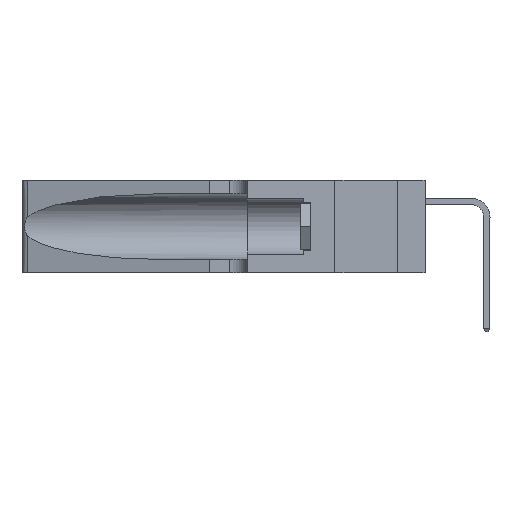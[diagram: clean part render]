
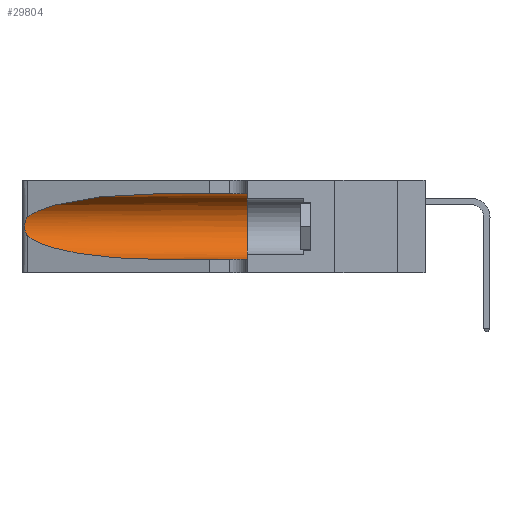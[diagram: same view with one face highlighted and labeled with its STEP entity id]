
A CAD part, left-side view. The second image highlights one B-rep face of the part: STEP entity #29804.
In plain terms, the highlighted cylindrical face has radius 3.308 mm (diameter 6.617 mm), a partial arc.
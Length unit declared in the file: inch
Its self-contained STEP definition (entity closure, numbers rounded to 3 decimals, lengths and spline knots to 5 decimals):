
#890 = EDGE_LOOP ( 'NONE', ( #8014, #15814, #40737, #19634, #7683, #2718 ) ) ;
#2718 = ORIENTED_EDGE ( 'NONE', *, *, #32880, .F. ) ;
#2881 = CARTESIAN_POINT ( 'NONE',  ( 0.25854, 1.2359, 0.20912 ) ) ;
#5132 = DIRECTION ( 'NONE',  ( 0., 1., 0. ) ) ;
#5824 = B_SPLINE_CURVE_WITH_KNOTS ( 'NONE', 3,
 ( #31138, #12391, #40559, #21838, #2881, #24994, #6144, #28142, #9344, #31278, #12522, #34421, #15643, #37551 ),
 .UNSPECIFIED., .F., .F.,
 ( 4, 2, 2, 2, 2, 2, 4 ),
 ( 0., 0.00027, 0.00053, 0.00107, 0.0016, 0.00187, 0.00214 ),
 .UNSPECIFIED. ) ;
#6144 = CARTESIAN_POINT ( 'NONE',  ( 0.26075, 1.23896, 0.19203 ) ) ;
#6509 = CARTESIAN_POINT ( 'NONE',  ( 0.1305, 0.72297, 0.31525 ) ) ;
#7683 = ORIENTED_EDGE ( 'NONE', *, *, #18345, .F. ) ;
#8014 = ORIENTED_EDGE ( 'NONE', *, *, #11465, .T. ) ;
#8963 = VERTEX_POINT ( 'NONE', #27738 ) ;
#9344 = CARTESIAN_POINT ( 'NONE',  ( 0.26017, 1.23833, 0.17102 ) ) ;
#9986 = AXIS2_PLACEMENT_3D ( 'NONE', #21427, #40135, #27585 ) ;
#10746 = VECTOR ( 'NONE', #35834, 39.37008 ) ;
#11465 = EDGE_CURVE ( 'NONE', #8963, #37218, #15659, .T. ) ;
#11480 = CYLINDRICAL_SURFACE ( 'NONE', #9986, 0.13025 ) ;
#11822 = VERTEX_POINT ( 'NONE', #36669 ) ;
#12210 = AXIS2_PLACEMENT_3D ( 'NONE', #24014, #5132, #27145 ) ;
#12391 = CARTESIAN_POINT ( 'NONE',  ( 0.25555, 1.22994, 0.2215 ) ) ;
#12522 = CARTESIAN_POINT ( 'NONE',  ( 0.25789, 1.23486, 0.15765 ) ) ;
#12623 = EDGE_CURVE ( 'NONE', #37218, #17556, #5824, .T. ) ;
#12871 = CARTESIAN_POINT ( 'NONE',  ( 0.18966, 0.96281, 0.31525 ) ) ;
#13072 = DIRECTION ( 'NONE',  ( 0., -1., 0. ) ) ;
#14107 = CARTESIAN_POINT ( 'NONE',  ( 0.2373, 1.15595, 0.08982 ) ) ;
#15177 = LINE ( 'NONE', #31843, #23533 ) ;
#15261 = EDGE_CURVE ( 'NONE', #17556, #11822, #23716, .T. ) ;
#15643 = CARTESIAN_POINT ( 'NONE',  ( 0.25555, 1.22993, 0.14849 ) ) ;
#15659 =( BOUNDED_CURVE ( )  B_SPLINE_CURVE ( 3, ( #6509, #12871, #37895, #19170 ),
 .UNSPECIFIED., .F., .F. ) 
 B_SPLINE_CURVE_WITH_KNOTS ( ( 4, 4 ),
 ( 1.5708, 2.84003 ),
 .UNSPECIFIED. ) 
 CURVE ( )  GEOMETRIC_REPRESENTATION_ITEM ( )  RATIONAL_B_SPLINE_CURVE ( ( 1., 0.87, 0.87, 1. ) ) 
 REPRESENTATION_ITEM ( '' )  );
#15814 = ORIENTED_EDGE ( 'NONE', *, *, #12623, .T. ) ;
#16245 = CARTESIAN_POINT ( 'NONE',  ( 0.1305, 0.35, 0.05475 ) ) ;
#16416 = CARTESIAN_POINT ( 'NONE',  ( 0.1305, 0.35, 0.31525 ) ) ;
#17083 = LINE ( 'NONE', #29542, #10746 ) ;
#17229 = CARTESIAN_POINT ( 'NONE',  ( 0.1305, 0.72297, 0.05475 ) ) ;
#17556 = VERTEX_POINT ( 'NONE', #31972 ) ;
#18345 = EDGE_CURVE ( 'NONE', #37442, #22489, #18725, .T. ) ;
#18725 = CIRCLE ( 'NONE', #12210, 0.13025 ) ;
#19170 = CARTESIAN_POINT ( 'NONE',  ( 0.25487, 1.22718, 0.22369 ) ) ;
#19634 = ORIENTED_EDGE ( 'NONE', *, *, #24446, .T. ) ;
#21427 = CARTESIAN_POINT ( 'NONE',  ( 0.1305, 1.61858, 0.185 ) ) ;
#21838 = CARTESIAN_POINT ( 'NONE',  ( 0.25787, 1.23484, 0.2124 ) ) ;
#22489 = VERTEX_POINT ( 'NONE', #16245 ) ;
#23533 = VECTOR ( 'NONE', #13072, 39.37008 ) ;
#23716 =( BOUNDED_CURVE ( )  B_SPLINE_CURVE ( 3, ( #32858, #14107, #35999, #17229 ),
 .UNSPECIFIED., .F., .T. ) 
 B_SPLINE_CURVE_WITH_KNOTS ( ( 4, 4 ),
 ( 3.44316, 4.71239 ),
 .UNSPECIFIED. ) 
 CURVE ( )  GEOMETRIC_REPRESENTATION_ITEM ( )  RATIONAL_B_SPLINE_CURVE ( ( 1., 0.87, 0.87, 1. ) ) 
 REPRESENTATION_ITEM ( '' )  );
#24014 = CARTESIAN_POINT ( 'NONE',  ( 0.1305, 0.35, 0.185 ) ) ;
#24446 = EDGE_CURVE ( 'NONE', #11822, #22489, #17083, .T. ) ;
#24994 = CARTESIAN_POINT ( 'NONE',  ( 0.26018, 1.23835, 0.19895 ) ) ;
#27145 = DIRECTION ( 'NONE',  ( 0., 0., 1. ) ) ;
#27585 = DIRECTION ( 'NONE',  ( 0., 0., -1. ) ) ;
#27738 = CARTESIAN_POINT ( 'NONE',  ( 0.1305, 0.72297, 0.31525 ) ) ;
#28142 = CARTESIAN_POINT ( 'NONE',  ( 0.26075, 1.23896, 0.178 ) ) ;
#29542 = CARTESIAN_POINT ( 'NONE',  ( 0.1305, 1.61858, 0.05475 ) ) ;
#29804 = ADVANCED_FACE ( 'NONE', ( #36456 ), #11480, .F. ) ;
#31138 = CARTESIAN_POINT ( 'NONE',  ( 0.25487, 1.22718, 0.22369 ) ) ;
#31278 = CARTESIAN_POINT ( 'NONE',  ( 0.25856, 1.23593, 0.16098 ) ) ;
#31843 = CARTESIAN_POINT ( 'NONE',  ( 0.1305, 1.61858, 0.31525 ) ) ;
#31972 = CARTESIAN_POINT ( 'NONE',  ( 0.25487, 1.22718, 0.14631 ) ) ;
#32858 = CARTESIAN_POINT ( 'NONE',  ( 0.25487, 1.22718, 0.14631 ) ) ;
#32880 = EDGE_CURVE ( 'NONE', #8963, #37442, #15177, .T. ) ;
#33995 = CARTESIAN_POINT ( 'NONE',  ( 0.25487, 1.22718, 0.22369 ) ) ;
#34421 = CARTESIAN_POINT ( 'NONE',  ( 0.25639, 1.23186, 0.15144 ) ) ;
#35834 = DIRECTION ( 'NONE',  ( 0., -1., 0. ) ) ;
#35999 = CARTESIAN_POINT ( 'NONE',  ( 0.18966, 0.96281, 0.05475 ) ) ;
#36456 = FACE_OUTER_BOUND ( 'NONE', #890, .T. ) ;
#36669 = CARTESIAN_POINT ( 'NONE',  ( 0.1305, 0.72297, 0.05475 ) ) ;
#37218 = VERTEX_POINT ( 'NONE', #33995 ) ;
#37442 = VERTEX_POINT ( 'NONE', #16416 ) ;
#37551 = CARTESIAN_POINT ( 'NONE',  ( 0.25487, 1.22718, 0.14631 ) ) ;
#37895 = CARTESIAN_POINT ( 'NONE',  ( 0.2373, 1.15595, 0.28018 ) ) ;
#40135 = DIRECTION ( 'NONE',  ( 0., -1., 0. ) ) ;
#40559 = CARTESIAN_POINT ( 'NONE',  ( 0.25639, 1.23184, 0.21858 ) ) ;
#40737 = ORIENTED_EDGE ( 'NONE', *, *, #15261, .T. ) ;
